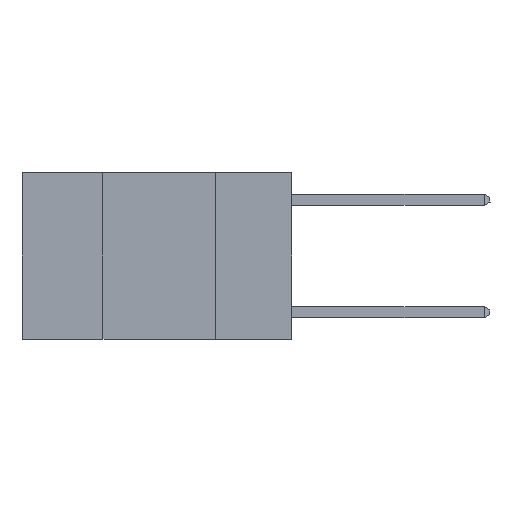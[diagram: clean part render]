
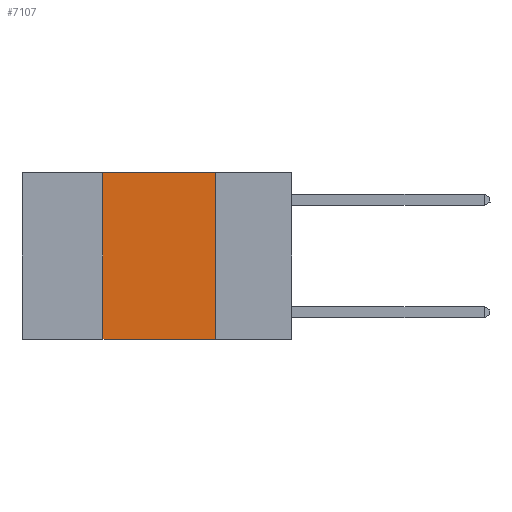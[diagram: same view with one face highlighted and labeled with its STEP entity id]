
A CAD part, left-side view. The second image highlights one B-rep face of the part: STEP entity #7107.
In plain terms, the highlighted planar face has unit normal (-1, 0, 0).
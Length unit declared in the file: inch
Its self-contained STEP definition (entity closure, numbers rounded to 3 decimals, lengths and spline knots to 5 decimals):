
#175 = DIRECTION ( 'NONE',  ( 0., -1., 0. ) ) ;
#1089 = CARTESIAN_POINT ( 'NONE',  ( 0., 0.17, 0. ) ) ;
#1169 = AXIS2_PLACEMENT_3D ( 'NONE', #13958, #5902, #15321 ) ;
#1589 = ORIENTED_EDGE ( 'NONE', *, *, #15480, .F. ) ;
#1834 = PLANE ( 'NONE',  #1169 ) ;
#2373 = FACE_OUTER_BOUND ( 'NONE', #10282, .T. ) ;
#2470 = CARTESIAN_POINT ( 'NONE',  ( 0., 0.42, 0. ) ) ;
#3105 = EDGE_CURVE ( 'NONE', #15504, #15459, #7737, .T. ) ;
#4061 = EDGE_CURVE ( 'NONE', #15303, #15504, #13201, .T. ) ;
#4310 = DIRECTION ( 'NONE',  ( 0., 0., 1. ) ) ;
#4582 = VERTEX_POINT ( 'NONE', #9493 ) ;
#4947 = ORIENTED_EDGE ( 'NONE', *, *, #5034, .T. ) ;
#5034 = EDGE_CURVE ( 'NONE', #4582, #15459, #12289, .T. ) ;
#5668 = CARTESIAN_POINT ( 'NONE',  ( 0., 0.17, 0. ) ) ;
#5902 = DIRECTION ( 'NONE',  ( 1., 0., 0. ) ) ;
#6126 = LINE ( 'NONE', #8266, #12818 ) ;
#7107 = ADVANCED_FACE ( 'NONE', ( #2373 ), #1834, .F. ) ;
#7132 = CARTESIAN_POINT ( 'NONE',  ( 0., 0.6, 0. ) ) ;
#7737 = LINE ( 'NONE', #1089, #13654 ) ;
#8266 = CARTESIAN_POINT ( 'NONE',  ( 0., 0.42, 0. ) ) ;
#8423 = ORIENTED_EDGE ( 'NONE', *, *, #4061, .F. ) ;
#8462 = DIRECTION ( 'NONE',  ( 0., -1., 0. ) ) ;
#8696 = VECTOR ( 'NONE', #175, 39.37008 ) ;
#9493 = CARTESIAN_POINT ( 'NONE',  ( 0., 0.42, -0.37 ) ) ;
#9990 = VECTOR ( 'NONE', #8462, 39.37008 ) ;
#10282 = EDGE_LOOP ( 'NONE', ( #17033, #8423, #1589, #4947 ) ) ;
#12289 = LINE ( 'NONE', #16281, #8696 ) ;
#12818 = VECTOR ( 'NONE', #4310, 39.37008 ) ;
#13201 = LINE ( 'NONE', #7132, #9990 ) ;
#13654 = VECTOR ( 'NONE', #15807, 39.37008 ) ;
#13958 = CARTESIAN_POINT ( 'NONE',  ( 0., 0.6, 0. ) ) ;
#15019 = CARTESIAN_POINT ( 'NONE',  ( 0., 0.17, -0.37 ) ) ;
#15303 = VERTEX_POINT ( 'NONE', #2470 ) ;
#15321 = DIRECTION ( 'NONE',  ( 0., 0., -1. ) ) ;
#15459 = VERTEX_POINT ( 'NONE', #15019 ) ;
#15480 = EDGE_CURVE ( 'NONE', #4582, #15303, #6126, .T. ) ;
#15504 = VERTEX_POINT ( 'NONE', #5668 ) ;
#15807 = DIRECTION ( 'NONE',  ( 0., 0., -1. ) ) ;
#16281 = CARTESIAN_POINT ( 'NONE',  ( 0., 0.6, -0.37 ) ) ;
#17033 = ORIENTED_EDGE ( 'NONE', *, *, #3105, .F. ) ;
